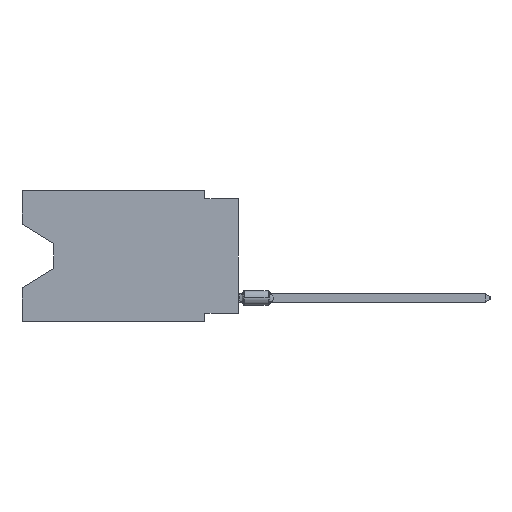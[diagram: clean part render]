
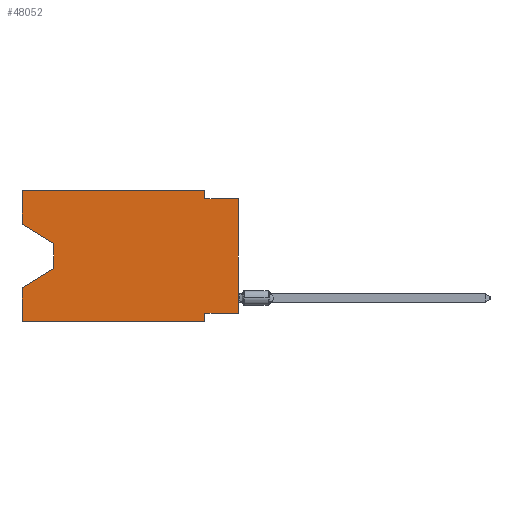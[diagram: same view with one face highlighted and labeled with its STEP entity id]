
A CAD part, left-side view. The second image highlights one B-rep face of the part: STEP entity #48052.
In plain terms, the highlighted planar face has unit normal (-1, 0, 0).
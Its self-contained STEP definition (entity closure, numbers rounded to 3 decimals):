
#2258 = CARTESIAN_POINT ( 'NONE',  ( 0., 16.383, -9.906 ) ) ;
#2628 = VECTOR ( 'NONE', #12002, 1000. ) ;
#2948 = CARTESIAN_POINT ( 'NONE',  ( 0., 0., -0.635 ) ) ;
#3156 = VERTEX_POINT ( 'NONE', #10920 ) ;
#3475 = PLANE ( 'NONE',  #44026 ) ;
#3788 = CARTESIAN_POINT ( 'NONE',  ( 0., 0., -0.635 ) ) ;
#3922 = CARTESIAN_POINT ( 'NONE',  ( 0., 2.54, -9.906 ) ) ;
#5548 = DIRECTION ( 'NONE',  ( 0., -0.855, -0.519 ) ) ;
#5581 = LINE ( 'NONE', #37225, #24367 ) ;
#6556 = EDGE_CURVE ( 'NONE', #17758, #13890, #33656, .T. ) ;
#7167 = EDGE_CURVE ( 'NONE', #19518, #44156, #22369, .T. ) ;
#7818 = CARTESIAN_POINT ( 'NONE',  ( 0., 2.54, 0. ) ) ;
#8258 = ORIENTED_EDGE ( 'NONE', *, *, #14269, .F. ) ;
#8432 = ORIENTED_EDGE ( 'NONE', *, *, #13567, .T. ) ;
#9127 = CARTESIAN_POINT ( 'NONE',  ( 0., 16.383, 0. ) ) ;
#10318 = CARTESIAN_POINT ( 'NONE',  ( 0., 16.383, -2.546 ) ) ;
#10920 = CARTESIAN_POINT ( 'NONE',  ( 0., 13.97, -5.893 ) ) ;
#11184 = CARTESIAN_POINT ( 'NONE',  ( 0., 16.383, 0. ) ) ;
#12002 = DIRECTION ( 'NONE',  ( 0., 0., 1. ) ) ;
#12396 = DIRECTION ( 'NONE',  ( 0., -1., 0. ) ) ;
#12441 = DIRECTION ( 'NONE',  ( 0., 0.855, -0.519 ) ) ;
#12705 = LINE ( 'NONE', #32934, #41469 ) ;
#12839 = DIRECTION ( 'NONE',  ( 0., -1., 0. ) ) ;
#13338 = VERTEX_POINT ( 'NONE', #51011 ) ;
#13567 = EDGE_CURVE ( 'NONE', #28365, #40804, #12705, .T. ) ;
#13759 = ORIENTED_EDGE ( 'NONE', *, *, #7167, .F. ) ;
#13890 = VERTEX_POINT ( 'NONE', #3922 ) ;
#13951 = VECTOR ( 'NONE', #12441, 1000. ) ;
#14269 = EDGE_CURVE ( 'NONE', #17758, #19656, #43197, .T. ) ;
#15831 = EDGE_CURVE ( 'NONE', #13338, #44156, #32740, .T. ) ;
#16276 = DIRECTION ( 'NONE',  ( 0., 0., -1. ) ) ;
#17758 = VERTEX_POINT ( 'NONE', #2258 ) ;
#17829 = LINE ( 'NONE', #50476, #45398 ) ;
#17932 = EDGE_CURVE ( 'NONE', #36523, #19518, #17829, .T. ) ;
#18262 = EDGE_CURVE ( 'NONE', #3156, #19656, #36658, .T. ) ;
#19518 = VERTEX_POINT ( 'NONE', #21881 ) ;
#19565 = LINE ( 'NONE', #27268, #43200 ) ;
#19656 = VERTEX_POINT ( 'NONE', #47344 ) ;
#19963 = DIRECTION ( 'NONE',  ( 1., 0., 0. ) ) ;
#20294 = CARTESIAN_POINT ( 'NONE',  ( 0., 2.54, -9.271 ) ) ;
#20502 = VECTOR ( 'NONE', #49532, 1000. ) ;
#21408 = LINE ( 'NONE', #45828, #20502 ) ;
#21881 = CARTESIAN_POINT ( 'NONE',  ( 0., 2.54, -0.635 ) ) ;
#22369 = LINE ( 'NONE', #2948, #42481 ) ;
#22644 = ORIENTED_EDGE ( 'NONE', *, *, #6556, .T. ) ;
#23410 = VECTOR ( 'NONE', #12839, 1000. ) ;
#24367 = VECTOR ( 'NONE', #34010, 1000. ) ;
#25701 = EDGE_CURVE ( 'NONE', #40804, #3156, #5581, .T. ) ;
#26875 = DIRECTION ( 'NONE',  ( 0., 0., -1. ) ) ;
#27251 = DIRECTION ( 'NONE',  ( 0., 0., 1. ) ) ;
#27268 = CARTESIAN_POINT ( 'NONE',  ( 0., 16.383, 0. ) ) ;
#27707 = CARTESIAN_POINT ( 'NONE',  ( 0., 0., 0. ) ) ;
#28365 = VERTEX_POINT ( 'NONE', #10318 ) ;
#29415 = CARTESIAN_POINT ( 'NONE',  ( 0., 16.383, -9.906 ) ) ;
#29472 = VERTEX_POINT ( 'NONE', #20294 ) ;
#30662 = EDGE_CURVE ( 'NONE', #29472, #13890, #32513, .T. ) ;
#31344 = ORIENTED_EDGE ( 'NONE', *, *, #15831, .T. ) ;
#31467 = CARTESIAN_POINT ( 'NONE',  ( 0., 16.383, 0. ) ) ;
#31520 = CARTESIAN_POINT ( 'NONE',  ( 0., 16.383, 0. ) ) ;
#31645 = VECTOR ( 'NONE', #16276, 1000. ) ;
#32513 = LINE ( 'NONE', #44961, #31645 ) ;
#32740 = LINE ( 'NONE', #27707, #2628 ) ;
#32934 = CARTESIAN_POINT ( 'NONE',  ( 0., 16.383, -2.546 ) ) ;
#33005 = EDGE_CURVE ( 'NONE', #28365, #51617, #19565, .T. ) ;
#33656 = LINE ( 'NONE', #29415, #49202 ) ;
#34010 = DIRECTION ( 'NONE',  ( 0., 0., -1. ) ) ;
#34806 = ORIENTED_EDGE ( 'NONE', *, *, #35063, .F. ) ;
#35063 = EDGE_CURVE ( 'NONE', #13338, #29472, #21408, .T. ) ;
#36224 = EDGE_LOOP ( 'NONE', ( #8432, #47816, #37054, #8258, #22644, #51399, #34806, #31344, #13759, #43001, #43824, #49302 ) ) ;
#36523 = VERTEX_POINT ( 'NONE', #7818 ) ;
#36658 = LINE ( 'NONE', #45654, #13951 ) ;
#37045 = CARTESIAN_POINT ( 'NONE',  ( 0., 13.97, -4.013 ) ) ;
#37054 = ORIENTED_EDGE ( 'NONE', *, *, #18262, .T. ) ;
#37225 = CARTESIAN_POINT ( 'NONE',  ( 0., 13.97, -4.013 ) ) ;
#38591 = DIRECTION ( 'NONE',  ( 0., -1., 0. ) ) ;
#38820 = DIRECTION ( 'NONE',  ( 0., 0., -1. ) ) ;
#40034 = DIRECTION ( 'NONE',  ( 0., 0., 1. ) ) ;
#40635 = VECTOR ( 'NONE', #27251, 1000. ) ;
#40804 = VERTEX_POINT ( 'NONE', #37045 ) ;
#41307 = LINE ( 'NONE', #9127, #23410 ) ;
#41469 = VECTOR ( 'NONE', #5548, 1000. ) ;
#42481 = VECTOR ( 'NONE', #38591, 1000. ) ;
#43001 = ORIENTED_EDGE ( 'NONE', *, *, #17932, .F. ) ;
#43197 = LINE ( 'NONE', #31520, #40635 ) ;
#43200 = VECTOR ( 'NONE', #40034, 1000. ) ;
#43824 = ORIENTED_EDGE ( 'NONE', *, *, #46137, .F. ) ;
#44026 = AXIS2_PLACEMENT_3D ( 'NONE', #11184, #19963, #26875 ) ;
#44156 = VERTEX_POINT ( 'NONE', #3788 ) ;
#44961 = CARTESIAN_POINT ( 'NONE',  ( 0., 2.54, -9.906 ) ) ;
#45398 = VECTOR ( 'NONE', #38820, 1000. ) ;
#45654 = CARTESIAN_POINT ( 'NONE',  ( 0., 13.97, -5.893 ) ) ;
#45828 = CARTESIAN_POINT ( 'NONE',  ( 0., 0., -9.271 ) ) ;
#46137 = EDGE_CURVE ( 'NONE', #51617, #36523, #41307, .T. ) ;
#47344 = CARTESIAN_POINT ( 'NONE',  ( 0., 16.383, -7.36 ) ) ;
#47816 = ORIENTED_EDGE ( 'NONE', *, *, #25701, .T. ) ;
#48052 = ADVANCED_FACE ( 'NONE', ( #51297 ), #3475, .F. ) ;
#49202 = VECTOR ( 'NONE', #12396, 1000. ) ;
#49302 = ORIENTED_EDGE ( 'NONE', *, *, #33005, .F. ) ;
#49532 = DIRECTION ( 'NONE',  ( 0., 1., 0. ) ) ;
#50476 = CARTESIAN_POINT ( 'NONE',  ( 0., 2.54, 0. ) ) ;
#51011 = CARTESIAN_POINT ( 'NONE',  ( 0., 0., -9.271 ) ) ;
#51297 = FACE_OUTER_BOUND ( 'NONE', #36224, .T. ) ;
#51399 = ORIENTED_EDGE ( 'NONE', *, *, #30662, .F. ) ;
#51617 = VERTEX_POINT ( 'NONE', #31467 ) ;
